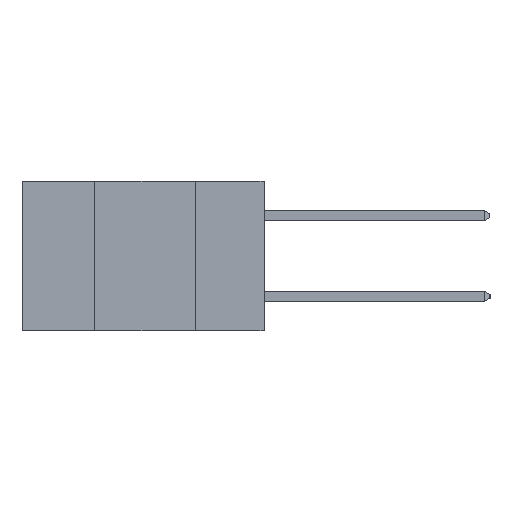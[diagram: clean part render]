
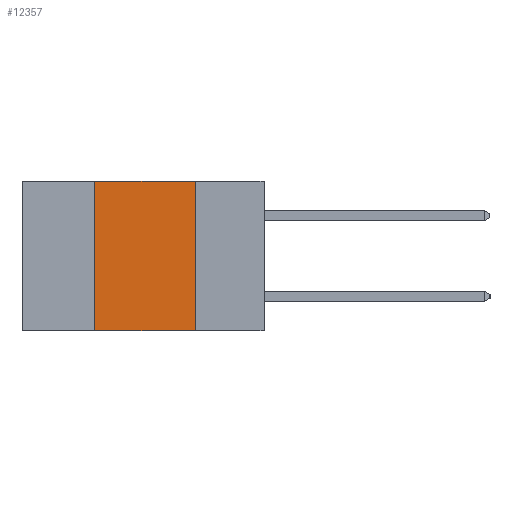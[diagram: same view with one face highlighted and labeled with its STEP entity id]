
A CAD part, left-side view. The second image highlights one B-rep face of the part: STEP entity #12357.
In plain terms, the highlighted planar face has unit normal (-1, 0, 0).
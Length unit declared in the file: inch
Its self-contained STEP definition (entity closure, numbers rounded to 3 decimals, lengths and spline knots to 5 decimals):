
#112 = ORIENTED_EDGE ( 'NONE', *, *, #2493, .F. ) ;
#1134 = CARTESIAN_POINT ( 'NONE',  ( 0., 0.42, 0. ) ) ;
#1351 = VERTEX_POINT ( 'NONE', #1134 ) ;
#1524 = VERTEX_POINT ( 'NONE', #12203 ) ;
#1709 = LINE ( 'NONE', #10478, #9540 ) ;
#1898 = EDGE_CURVE ( 'NONE', #8923, #1524, #11960, .T. ) ;
#2026 = DIRECTION ( 'NONE',  ( 1., 0., 0. ) ) ;
#2341 = ORIENTED_EDGE ( 'NONE', *, *, #1898, .F. ) ;
#2421 = EDGE_LOOP ( 'NONE', ( #2341, #5505, #112, #3365 ) ) ;
#2493 = EDGE_CURVE ( 'NONE', #9385, #1351, #11006, .T. ) ;
#2748 = FACE_OUTER_BOUND ( 'NONE', #2421, .T. ) ;
#2881 = CARTESIAN_POINT ( 'NONE',  ( 0., 0.17, 0. ) ) ;
#3359 = EDGE_CURVE ( 'NONE', #1351, #8923, #1709, .T. ) ;
#3365 = ORIENTED_EDGE ( 'NONE', *, *, #4050, .T. ) ;
#4050 = EDGE_CURVE ( 'NONE', #9385, #1524, #5678, .T. ) ;
#4276 = VECTOR ( 'NONE', #10748, 39.37008 ) ;
#5390 = DIRECTION ( 'NONE',  ( 0., 0., 1. ) ) ;
#5505 = ORIENTED_EDGE ( 'NONE', *, *, #3359, .F. ) ;
#5678 = LINE ( 'NONE', #12443, #10247 ) ;
#5819 = CARTESIAN_POINT ( 'NONE',  ( 0., 0.42, -0.37 ) ) ;
#6016 = CARTESIAN_POINT ( 'NONE',  ( 0., 0.42, -0.37 ) ) ;
#6159 = CARTESIAN_POINT ( 'NONE',  ( 0., 0.6, 0. ) ) ;
#8208 = PLANE ( 'NONE',  #12661 ) ;
#8923 = VERTEX_POINT ( 'NONE', #2881 ) ;
#9175 = DIRECTION ( 'NONE',  ( 0., 0., -1. ) ) ;
#9385 = VERTEX_POINT ( 'NONE', #6016 ) ;
#9540 = VECTOR ( 'NONE', #10814, 39.37008 ) ;
#10247 = VECTOR ( 'NONE', #11750, 39.37008 ) ;
#10437 = VECTOR ( 'NONE', #5390, 39.37008 ) ;
#10478 = CARTESIAN_POINT ( 'NONE',  ( 0., 0.6, 0. ) ) ;
#10748 = DIRECTION ( 'NONE',  ( 0., 0., -1. ) ) ;
#10814 = DIRECTION ( 'NONE',  ( 0., -1., 0. ) ) ;
#11006 = LINE ( 'NONE', #5819, #10437 ) ;
#11033 = CARTESIAN_POINT ( 'NONE',  ( 0., 0.17, -0.37 ) ) ;
#11750 = DIRECTION ( 'NONE',  ( 0., -1., 0. ) ) ;
#11960 = LINE ( 'NONE', #11033, #4276 ) ;
#12203 = CARTESIAN_POINT ( 'NONE',  ( 0., 0.17, -0.37 ) ) ;
#12357 = ADVANCED_FACE ( 'NONE', ( #2748 ), #8208, .F. ) ;
#12443 = CARTESIAN_POINT ( 'NONE',  ( 0., 0.6, -0.37 ) ) ;
#12661 = AXIS2_PLACEMENT_3D ( 'NONE', #6159, #2026, #9175 ) ;
